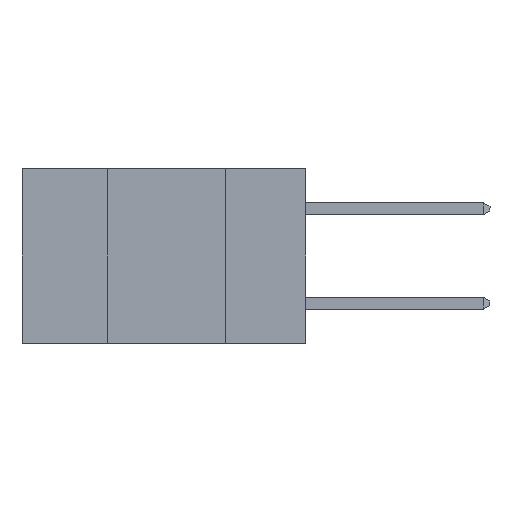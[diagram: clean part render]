
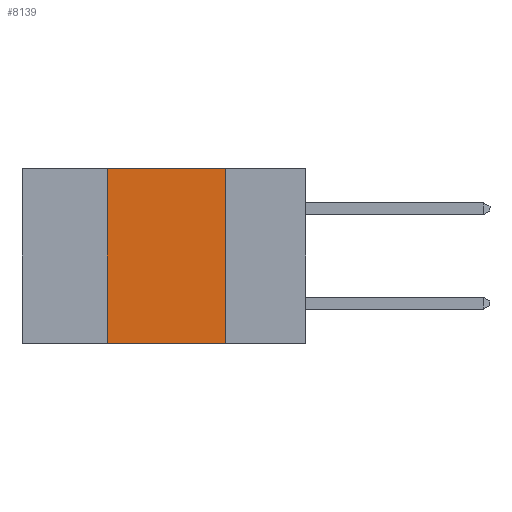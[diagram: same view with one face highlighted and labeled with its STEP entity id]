
A CAD part, left-side view. The second image highlights one B-rep face of the part: STEP entity #8139.
In plain terms, the highlighted planar face has unit normal (-1, 0, 0).
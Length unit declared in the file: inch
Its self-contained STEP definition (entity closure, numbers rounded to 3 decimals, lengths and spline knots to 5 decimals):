
#109 = ORIENTED_EDGE ( 'NONE', *, *, #1725, .T. ) ;
#130 = CARTESIAN_POINT ( 'NONE',  ( 0., 0.42, -0.37 ) ) ;
#551 = VERTEX_POINT ( 'NONE', #130 ) ;
#570 = VECTOR ( 'NONE', #7238, 39.37008 ) ;
#1061 = ORIENTED_EDGE ( 'NONE', *, *, #1280, .F. ) ;
#1114 = CARTESIAN_POINT ( 'NONE',  ( 0., 0.17, -0.37 ) ) ;
#1225 = AXIS2_PLACEMENT_3D ( 'NONE', #5227, #2903, #5319 ) ;
#1280 = EDGE_CURVE ( 'NONE', #551, #2995, #1412, .T. ) ;
#1412 = LINE ( 'NONE', #4352, #570 ) ;
#1541 = CARTESIAN_POINT ( 'NONE',  ( 0., 0.17, -0.37 ) ) ;
#1631 = VECTOR ( 'NONE', #8025, 39.37008 ) ;
#1725 = EDGE_CURVE ( 'NONE', #551, #6524, #7783, .T. ) ;
#1773 = EDGE_CURVE ( 'NONE', #8396, #6524, #5125, .T. ) ;
#2141 = DIRECTION ( 'NONE',  ( 0., -1., 0. ) ) ;
#2182 = DIRECTION ( 'NONE',  ( 0., 0., -1. ) ) ;
#2247 = CARTESIAN_POINT ( 'NONE',  ( 0., 0.42, 0. ) ) ;
#2903 = DIRECTION ( 'NONE',  ( 1., 0., 0. ) ) ;
#2995 = VERTEX_POINT ( 'NONE', #2247 ) ;
#3221 = CARTESIAN_POINT ( 'NONE',  ( 0., 0.17, 0. ) ) ;
#4337 = CARTESIAN_POINT ( 'NONE',  ( 0., 0.6, -0.37 ) ) ;
#4352 = CARTESIAN_POINT ( 'NONE',  ( 0., 0.42, -0.37 ) ) ;
#4386 = EDGE_CURVE ( 'NONE', #2995, #8396, #7980, .T. ) ;
#4589 = CARTESIAN_POINT ( 'NONE',  ( 0., 0.6, 0. ) ) ;
#4776 = ORIENTED_EDGE ( 'NONE', *, *, #1773, .F. ) ;
#5125 = LINE ( 'NONE', #1541, #8608 ) ;
#5227 = CARTESIAN_POINT ( 'NONE',  ( 0., 0.6, 0. ) ) ;
#5319 = DIRECTION ( 'NONE',  ( 0., 0., -1. ) ) ;
#5923 = PLANE ( 'NONE',  #1225 ) ;
#5944 = EDGE_LOOP ( 'NONE', ( #4776, #6134, #1061, #109 ) ) ;
#6134 = ORIENTED_EDGE ( 'NONE', *, *, #4386, .F. ) ;
#6524 = VERTEX_POINT ( 'NONE', #1114 ) ;
#7149 = FACE_OUTER_BOUND ( 'NONE', #5944, .T. ) ;
#7238 = DIRECTION ( 'NONE',  ( 0., 0., 1. ) ) ;
#7573 = VECTOR ( 'NONE', #2141, 39.37008 ) ;
#7783 = LINE ( 'NONE', #4337, #7573 ) ;
#7980 = LINE ( 'NONE', #4589, #1631 ) ;
#8025 = DIRECTION ( 'NONE',  ( 0., -1., 0. ) ) ;
#8139 = ADVANCED_FACE ( 'NONE', ( #7149 ), #5923, .F. ) ;
#8396 = VERTEX_POINT ( 'NONE', #3221 ) ;
#8608 = VECTOR ( 'NONE', #2182, 39.37008 ) ;
